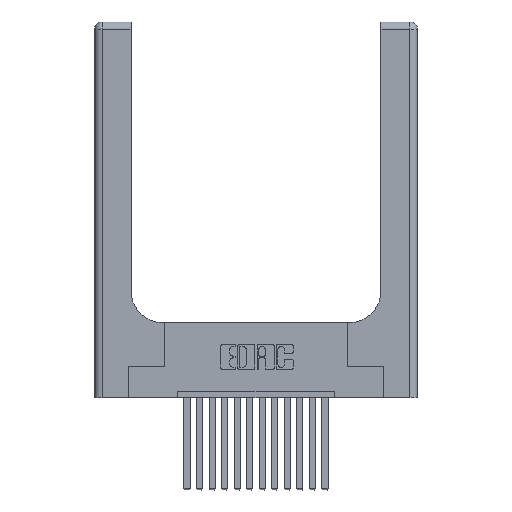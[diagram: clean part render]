
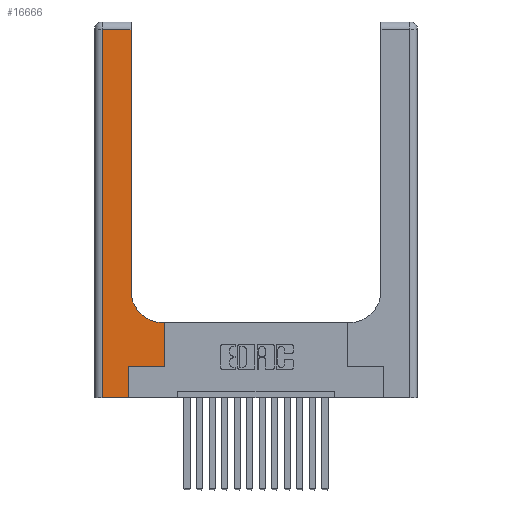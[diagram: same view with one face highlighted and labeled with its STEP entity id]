
A CAD part, top view. The second image highlights one B-rep face of the part: STEP entity #16666.
In plain terms, the highlighted planar face has unit normal (0, 0, 1).
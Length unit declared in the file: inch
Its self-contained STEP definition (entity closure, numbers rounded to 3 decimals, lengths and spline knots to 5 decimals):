
#397 = CARTESIAN_POINT ( 'NONE',  ( 0.5585, 0.25, 0.37 ) ) ;
#459 = LINE ( 'NONE', #7013, #13539 ) ;
#1380 = CARTESIAN_POINT ( 'NONE',  ( 0.269, 0.25, 0.37 ) ) ;
#1463 = CARTESIAN_POINT ( 'NONE',  ( 0.06, 2.94, 0.37 ) ) ;
#1544 = AXIS2_PLACEMENT_3D ( 'NONE', #8027, #14108, #13746 ) ;
#2285 = VERTEX_POINT ( 'NONE', #1380 ) ;
#2293 = CARTESIAN_POINT ( 'NONE',  ( 0.5585, 0.25, 0.37 ) ) ;
#2965 = CARTESIAN_POINT ( 'NONE',  ( 0.2915, 0.6, 0.37 ) ) ;
#3088 = CARTESIAN_POINT ( 'NONE',  ( 0.06, 0., 0.37 ) ) ;
#3182 = EDGE_CURVE ( 'NONE', #8600, #7222, #5456, .T. ) ;
#3759 = ORIENTED_EDGE ( 'NONE', *, *, #11561, .T. ) ;
#4373 = DIRECTION ( 'NONE',  ( 0., 0., -1. ) ) ;
#4766 = VECTOR ( 'NONE', #17437, 39.37008 ) ;
#5246 = ORIENTED_EDGE ( 'NONE', *, *, #8394, .T. ) ;
#5298 = CARTESIAN_POINT ( 'NONE',  ( 0.5415, 0.6, 0.37 ) ) ;
#5311 = VECTOR ( 'NONE', #8737, 39.37008 ) ;
#5456 = LINE ( 'NONE', #2293, #6315 ) ;
#5523 = FACE_OUTER_BOUND ( 'NONE', #14595, .T. ) ;
#5624 = CARTESIAN_POINT ( 'NONE',  ( 0., 3., 0.37 ) ) ;
#5654 = CARTESIAN_POINT ( 'NONE',  ( 0.2915, 3., 0.37 ) ) ;
#5712 = ORIENTED_EDGE ( 'NONE', *, *, #11173, .T. ) ;
#5867 = VECTOR ( 'NONE', #8515, 39.37008 ) ;
#5911 = CARTESIAN_POINT ( 'NONE',  ( 0.269, 0., 0.37 ) ) ;
#6315 = VECTOR ( 'NONE', #11992, 39.37008 ) ;
#6382 = VERTEX_POINT ( 'NONE', #15224 ) ;
#6870 = EDGE_CURVE ( 'NONE', #10787, #2285, #10341, .T. ) ;
#7013 = CARTESIAN_POINT ( 'NONE',  ( 0.06, 3., 0.37 ) ) ;
#7159 = VERTEX_POINT ( 'NONE', #1463 ) ;
#7222 = VERTEX_POINT ( 'NONE', #12672 ) ;
#8027 = CARTESIAN_POINT ( 'NONE',  ( 0.5415, 0.85, 0.37 ) ) ;
#8394 = EDGE_CURVE ( 'NONE', #7159, #14451, #459, .T. ) ;
#8515 = DIRECTION ( 'NONE',  ( -1., 0., 0. ) ) ;
#8600 = VERTEX_POINT ( 'NONE', #397 ) ;
#8737 = DIRECTION ( 'NONE',  ( 0., 1., 0. ) ) ;
#9134 = CARTESIAN_POINT ( 'NONE',  ( 0.269, 0.25, 0.37 ) ) ;
#9388 = ORIENTED_EDGE ( 'NONE', *, *, #6870, .T. ) ;
#9998 = VECTOR ( 'NONE', #16831, 39.37008 ) ;
#10290 = ORIENTED_EDGE ( 'NONE', *, *, #3182, .T. ) ;
#10341 = LINE ( 'NONE', #17377, #5311 ) ;
#10460 = EDGE_CURVE ( 'NONE', #2285, #8600, #17226, .T. ) ;
#10787 = VERTEX_POINT ( 'NONE', #5911 ) ;
#11128 = PLANE ( 'NONE',  #16250 ) ;
#11173 = EDGE_CURVE ( 'NONE', #7222, #17680, #17642, .T. ) ;
#11201 = DIRECTION ( 'NONE',  ( 0., -1., 0. ) ) ;
#11561 = EDGE_CURVE ( 'NONE', #6382, #17691, #12852, .T. ) ;
#11992 = DIRECTION ( 'NONE',  ( 0., 1., 0. ) ) ;
#12023 = EDGE_CURVE ( 'NONE', #17691, #7159, #15885, .T. ) ;
#12068 = CARTESIAN_POINT ( 'NONE',  ( 0.2915, 2.94, 0.37 ) ) ;
#12126 = ORIENTED_EDGE ( 'NONE', *, *, #10460, .T. ) ;
#12371 = CIRCLE ( 'NONE', #1544, 0.25 ) ;
#12549 = EDGE_CURVE ( 'NONE', #14451, #10787, #18034, .T. ) ;
#12672 = CARTESIAN_POINT ( 'NONE',  ( 0.5585, 0.6, 0.37 ) ) ;
#12852 = LINE ( 'NONE', #5654, #9998 ) ;
#12909 = EDGE_CURVE ( 'NONE', #17680, #6382, #12371, .T. ) ;
#13539 = VECTOR ( 'NONE', #11201, 39.37008 ) ;
#13546 = ORIENTED_EDGE ( 'NONE', *, *, #12023, .T. ) ;
#13746 = DIRECTION ( 'NONE',  ( 1., 0., 0. ) ) ;
#14108 = DIRECTION ( 'NONE',  ( 0., 0., -1. ) ) ;
#14113 = VECTOR ( 'NONE', #15085, 39.37008 ) ;
#14308 = VECTOR ( 'NONE', #16611, 39.37008 ) ;
#14451 = VERTEX_POINT ( 'NONE', #3088 ) ;
#14595 = EDGE_LOOP ( 'NONE', ( #3759, #13546, #5246, #15648, #9388, #12126, #10290, #5712, #16397 ) ) ;
#15085 = DIRECTION ( 'NONE',  ( -1., 0., 0. ) ) ;
#15224 = CARTESIAN_POINT ( 'NONE',  ( 0.2915, 0.85, 0.37 ) ) ;
#15648 = ORIENTED_EDGE ( 'NONE', *, *, #12549, .T. ) ;
#15885 = LINE ( 'NONE', #17955, #14113 ) ;
#16250 = AXIS2_PLACEMENT_3D ( 'NONE', #5624, #4373, #16682 ) ;
#16397 = ORIENTED_EDGE ( 'NONE', *, *, #12909, .T. ) ;
#16551 = CARTESIAN_POINT ( 'NONE',  ( 0., 0., 0.37 ) ) ;
#16611 = DIRECTION ( 'NONE',  ( 1., 0., 0. ) ) ;
#16666 = ADVANCED_FACE ( 'NONE', ( #5523 ), #11128, .F. ) ;
#16682 = DIRECTION ( 'NONE',  ( -1., 0., 0. ) ) ;
#16831 = DIRECTION ( 'NONE',  ( 0., 1., 0. ) ) ;
#17226 = LINE ( 'NONE', #9134, #4766 ) ;
#17377 = CARTESIAN_POINT ( 'NONE',  ( 0.269, 0., 0.37 ) ) ;
#17437 = DIRECTION ( 'NONE',  ( 1., 0., 0. ) ) ;
#17642 = LINE ( 'NONE', #2965, #5867 ) ;
#17680 = VERTEX_POINT ( 'NONE', #5298 ) ;
#17691 = VERTEX_POINT ( 'NONE', #12068 ) ;
#17955 = CARTESIAN_POINT ( 'NONE',  ( 0., 2.94, 0.37 ) ) ;
#18034 = LINE ( 'NONE', #16551, #14308 ) ;
